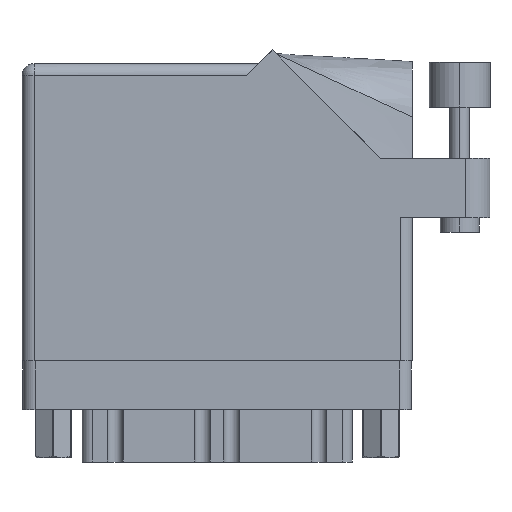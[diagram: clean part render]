
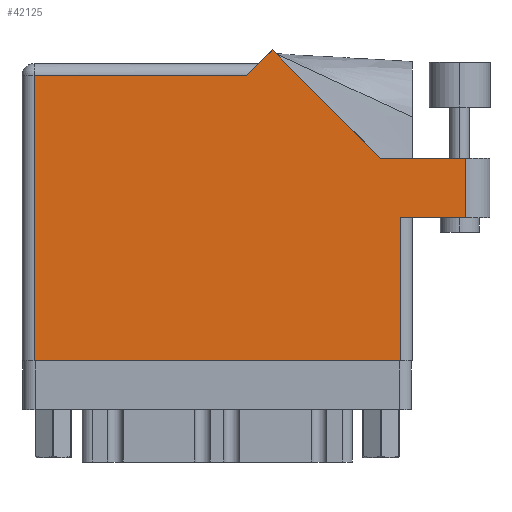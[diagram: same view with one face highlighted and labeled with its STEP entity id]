
A CAD part, front view. The second image highlights one B-rep face of the part: STEP entity #42125.
In plain terms, the highlighted face is planar.
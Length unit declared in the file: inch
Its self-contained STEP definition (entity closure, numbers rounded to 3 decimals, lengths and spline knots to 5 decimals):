
#1866 = CARTESIAN_POINT ( 'NONE',  ( 0.062, 0., 0. ) ) ;
#2252 = ORIENTED_EDGE ( 'NONE', *, *, #23037, .T. ) ;
#2743 = CARTESIAN_POINT ( 'NONE',  ( 1.84442, 1.044, 0. ) ) ;
#4088 = DIRECTION ( 'NONE',  ( 0., 1., 0. ) ) ;
#5525 = CARTESIAN_POINT ( 'NONE',  ( 2.41, 1.044, 0. ) ) ;
#5553 = VECTOR ( 'NONE', #9062, 39.37008 ) ;
#5855 = VECTOR ( 'NONE', #26254, 39.37008 ) ;
#5875 = EDGE_CURVE ( 'NONE', #43979, #47335, #12199, .T. ) ;
#6803 = DIRECTION ( 'NONE',  ( -0.707, 0.707, 0. ) ) ;
#6890 = ORIENTED_EDGE ( 'NONE', *, *, #5875, .T. ) ;
#7904 = EDGE_CURVE ( 'NONE', #17877, #20319, #28506, .T. ) ;
#8119 = CARTESIAN_POINT ( 'NONE',  ( 0.062, 0., 0. ) ) ;
#8365 = CARTESIAN_POINT ( 'NONE',  ( 0., 1.53, 0. ) ) ;
#9062 = DIRECTION ( 'NONE',  ( -1., 0., 0. ) ) ;
#10615 = ORIENTED_EDGE ( 'NONE', *, *, #38752, .T. ) ;
#11124 = DIRECTION ( 'NONE',  ( -0.707, -0.707, 0. ) ) ;
#11721 = VECTOR ( 'NONE', #19621, 39.37008 ) ;
#11984 = FACE_OUTER_BOUND ( 'NONE', #34379, .T. ) ;
#12199 = LINE ( 'NONE', #8119, #21806 ) ;
#12592 = AXIS2_PLACEMENT_3D ( 'NONE', #8365, #23048, #13880 ) ;
#13880 = DIRECTION ( 'NONE',  ( -1., 0., 0. ) ) ;
#15073 = CARTESIAN_POINT ( 'NONE',  ( 1.948, 0., 0. ) ) ;
#16257 = EDGE_CURVE ( 'NONE', #47335, #37508, #39998, .T. ) ;
#16515 = CARTESIAN_POINT ( 'NONE',  ( 1.28771, 1.60071, 0. ) ) ;
#16957 = CARTESIAN_POINT ( 'NONE',  ( 1.84442, 1.044, 0. ) ) ;
#17877 = VERTEX_POINT ( 'NONE', #47140 ) ;
#18732 = VERTEX_POINT ( 'NONE', #33643 ) ;
#19215 = LINE ( 'NONE', #26426, #39057 ) ;
#19621 = DIRECTION ( 'NONE',  ( 0., 1., 0. ) ) ;
#20319 = VERTEX_POINT ( 'NONE', #31870 ) ;
#20668 = CARTESIAN_POINT ( 'NONE',  ( 0.062, 1.468, 0. ) ) ;
#20896 = EDGE_CURVE ( 'NONE', #18732, #43693, #38913, .T. ) ;
#21806 = VECTOR ( 'NONE', #26865, 39.37008 ) ;
#21926 = ORIENTED_EDGE ( 'NONE', *, *, #20896, .T. ) ;
#23037 = EDGE_CURVE ( 'NONE', #43693, #34341, #28201, .T. ) ;
#23048 = DIRECTION ( 'NONE',  ( 0., 0., -1. ) ) ;
#23800 = DIRECTION ( 'NONE',  ( -1., 0., 0. ) ) ;
#23863 = VERTEX_POINT ( 'NONE', #33851 ) ;
#26254 = DIRECTION ( 'NONE',  ( 1., 0., 0. ) ) ;
#26297 = VECTOR ( 'NONE', #6803, 39.37008 ) ;
#26426 = CARTESIAN_POINT ( 'NONE',  ( 2.285, 1.044, 0. ) ) ;
#26651 = PLANE ( 'NONE',  #12592 ) ;
#26822 = CARTESIAN_POINT ( 'NONE',  ( 1.948, 0.737, 0. ) ) ;
#26865 = DIRECTION ( 'NONE',  ( 0., -1., 0. ) ) ;
#28201 = LINE ( 'NONE', #2743, #26297 ) ;
#28506 = LINE ( 'NONE', #31882, #5855 ) ;
#29427 = DIRECTION ( 'NONE',  ( 1., 0., 0. ) ) ;
#29859 = CARTESIAN_POINT ( 'NONE',  ( 1.217, 1.53, 0. ) ) ;
#29865 = ORIENTED_EDGE ( 'NONE', *, *, #41705, .T. ) ;
#30661 = LINE ( 'NONE', #26822, #11721 ) ;
#30917 = VECTOR ( 'NONE', #23800, 39.37008 ) ;
#31870 = CARTESIAN_POINT ( 'NONE',  ( 2.285, 0.737, 0. ) ) ;
#31882 = CARTESIAN_POINT ( 'NONE',  ( 2.01, 0.737, 0. ) ) ;
#32468 = EDGE_CURVE ( 'NONE', #20319, #18732, #19215, .T. ) ;
#33110 = ORIENTED_EDGE ( 'NONE', *, *, #32468, .T. ) ;
#33508 = CARTESIAN_POINT ( 'NONE',  ( 0., 0., 0. ) ) ;
#33643 = CARTESIAN_POINT ( 'NONE',  ( 2.285, 1.044, 0. ) ) ;
#33851 = CARTESIAN_POINT ( 'NONE',  ( 1.155, 1.468, 0. ) ) ;
#34341 = VERTEX_POINT ( 'NONE', #16515 ) ;
#34379 = EDGE_LOOP ( 'NONE', ( #44986, #33110, #21926, #2252, #29865, #42595, #6890, #34390, #10615 ) ) ;
#34390 = ORIENTED_EDGE ( 'NONE', *, *, #16257, .T. ) ;
#34537 = CARTESIAN_POINT ( 'NONE',  ( 0., 1.468, 0. ) ) ;
#37062 = LINE ( 'NONE', #29859, #44729 ) ;
#37508 = VERTEX_POINT ( 'NONE', #15073 ) ;
#37703 = EDGE_CURVE ( 'NONE', #23863, #43979, #38133, .T. ) ;
#38133 = LINE ( 'NONE', #34537, #5553 ) ;
#38752 = EDGE_CURVE ( 'NONE', #37508, #17877, #30661, .T. ) ;
#38913 = LINE ( 'NONE', #5525, #30917 ) ;
#39057 = VECTOR ( 'NONE', #4088, 39.37008 ) ;
#39998 = LINE ( 'NONE', #33508, #40267 ) ;
#40267 = VECTOR ( 'NONE', #29427, 39.37008 ) ;
#41705 = EDGE_CURVE ( 'NONE', #34341, #23863, #37062, .T. ) ;
#42125 = ADVANCED_FACE ( 'NONE', ( #11984 ), #26651, .F. ) ;
#42595 = ORIENTED_EDGE ( 'NONE', *, *, #37703, .T. ) ;
#43693 = VERTEX_POINT ( 'NONE', #16957 ) ;
#43979 = VERTEX_POINT ( 'NONE', #20668 ) ;
#44729 = VECTOR ( 'NONE', #11124, 39.37008 ) ;
#44986 = ORIENTED_EDGE ( 'NONE', *, *, #7904, .T. ) ;
#47140 = CARTESIAN_POINT ( 'NONE',  ( 1.948, 0.737, 0. ) ) ;
#47335 = VERTEX_POINT ( 'NONE', #1866 ) ;
